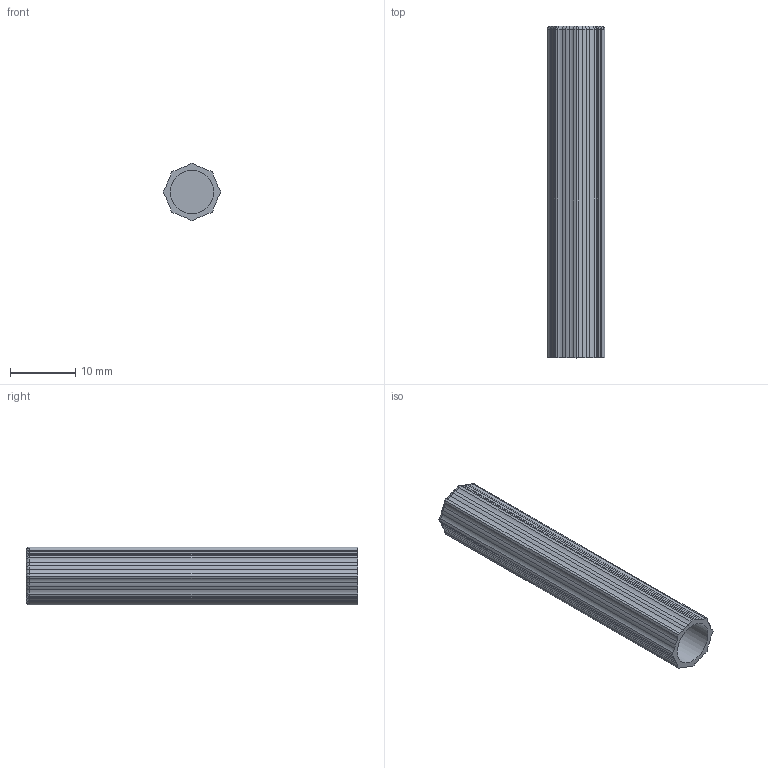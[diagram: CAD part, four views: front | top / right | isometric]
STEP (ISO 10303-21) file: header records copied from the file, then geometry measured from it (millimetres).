
FILE_DESCRIPTION(/* description */ (''),/* implementation_level */ '2;1');
FILE_NAME(/* name */ 'Chambering Insulator Inch (0.250in).stp',/* time_stamp */ '2021-02-15T01:56:46-06:00',/* author */ ('johne'),/* organization */ (''),/* preprocessor_version */ 'ST-DEVELOPER v18',/* originating_system */ 'Autodesk Inventor 2020',/* authorisation */ '');
FILE_SCHEMA (('AUTOMOTIVE_DESIGN { 1 0 10303 214 3 1 1 }'));
Length unit declared in the file: inch
Products named in the file (1): Chambering Insulator 250in rod
Bounding box: 8.82 x 50.8 x 8.82 mm (x, y, z)
Volume: 1049.3 mm3; surface area: 2493.3 mm2
Topology: 1 solids, 1 shells, 100 faces, 260 edges, 163 vertices
Faces by surface type: cylinder 49, torus 32, plane 19
Full cylindrical faces by diameter (mm): 6.629 x1
Entity records: 3402 total; most frequent: CARTESIAN_POINT 852, DIRECTION 561, ORIENTED_EDGE 520, EDGE_CURVE 260, AXIS2_PLACEMENT_3D 224, VERTEX_POINT 163, CIRCLE 115, LINE 113
